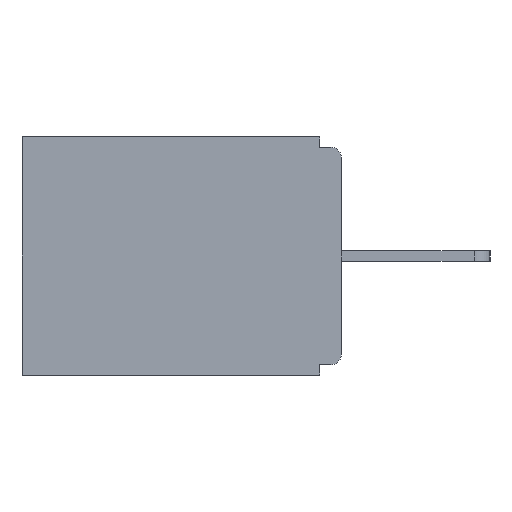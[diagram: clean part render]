
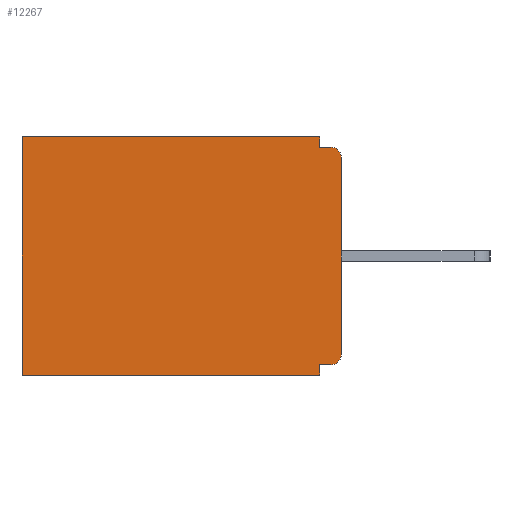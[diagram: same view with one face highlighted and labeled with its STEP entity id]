
A CAD part, left-side view. The second image highlights one B-rep face of the part: STEP entity #12267.
In plain terms, the highlighted planar face has unit normal (-1, 0, 0).
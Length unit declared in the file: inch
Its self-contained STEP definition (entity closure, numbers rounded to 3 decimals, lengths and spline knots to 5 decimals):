
#419 = DIRECTION ( 'NONE',  ( 0., 0., -1. ) ) ;
#435 = EDGE_CURVE ( 'NONE', #12971, #13632, #13769, .T. ) ;
#437 = VERTEX_POINT ( 'NONE', #7959 ) ;
#643 = CARTESIAN_POINT ( 'NONE',  ( 0.298, 0.015, -0.03 ) ) ;
#717 = DIRECTION ( 'NONE',  ( 0., -1., 0. ) ) ;
#756 = VERTEX_POINT ( 'NONE', #13736 ) ;
#789 = CARTESIAN_POINT ( 'NONE',  ( 0.298, 0.031, -0.328 ) ) ;
#1191 = VECTOR ( 'NONE', #7004, 39.37008 ) ;
#1245 = CIRCLE ( 'NONE', #14922, 0.015 ) ;
#1584 = CARTESIAN_POINT ( 'NONE',  ( 0.298, 0., -0.313 ) ) ;
#1650 = LINE ( 'NONE', #3609, #14662 ) ;
#1993 = EDGE_CURVE ( 'NONE', #756, #13632, #1245, .T. ) ;
#2159 = VERTEX_POINT ( 'NONE', #12462 ) ;
#2179 = CARTESIAN_POINT ( 'NONE',  ( 0.298, 0.031, -0.343 ) ) ;
#2371 = DIRECTION ( 'NONE',  ( 0., 1., 0. ) ) ;
#2685 = DIRECTION ( 'NONE',  ( 0., 0., -1. ) ) ;
#2760 = DIRECTION ( 'NONE',  ( -1., 0., 0. ) ) ;
#2870 = FACE_OUTER_BOUND ( 'NONE', #3330, .T. ) ;
#3187 = ORIENTED_EDGE ( 'NONE', *, *, #10290, .F. ) ;
#3330 = EDGE_LOOP ( 'NONE', ( #4592, #10694, #7637, #6819, #8735, #3187, #9320, #3805, #15769, #7374 ) ) ;
#3609 = CARTESIAN_POINT ( 'NONE',  ( 0.298, 0., -0.328 ) ) ;
#3805 = ORIENTED_EDGE ( 'NONE', *, *, #11930, .F. ) ;
#3869 = AXIS2_PLACEMENT_3D ( 'NONE', #14561, #7063, #15812 ) ;
#4266 = CARTESIAN_POINT ( 'NONE',  ( 0.298, 0.031, -0.343 ) ) ;
#4320 = DIRECTION ( 'NONE',  ( 0., 1., 0. ) ) ;
#4351 = VECTOR ( 'NONE', #5552, 39.37008 ) ;
#4395 = CARTESIAN_POINT ( 'NONE',  ( 0.298, 0., 0. ) ) ;
#4445 = CARTESIAN_POINT ( 'NONE',  ( 0.298, 0., -0.343 ) ) ;
#4592 = ORIENTED_EDGE ( 'NONE', *, *, #1993, .T. ) ;
#4597 = CARTESIAN_POINT ( 'NONE',  ( 0.298, 0., -0.015 ) ) ;
#4654 = LINE ( 'NONE', #14625, #1191 ) ;
#4920 = CARTESIAN_POINT ( 'NONE',  ( 0.298, 0.031, -0.343 ) ) ;
#5164 = CARTESIAN_POINT ( 'NONE',  ( 0.298, 0.015, -0.313 ) ) ;
#5245 = EDGE_CURVE ( 'NONE', #437, #15755, #4654, .T. ) ;
#5552 = DIRECTION ( 'NONE',  ( 0., 0., -1. ) ) ;
#5782 = PLANE ( 'NONE',  #3869 ) ;
#5918 = CARTESIAN_POINT ( 'NONE',  ( 0.298, 0.031, -0.015 ) ) ;
#6418 = VERTEX_POINT ( 'NONE', #4920 ) ;
#6627 = EDGE_CURVE ( 'NONE', #9645, #10092, #11172, .T. ) ;
#6661 = CARTESIAN_POINT ( 'NONE',  ( 0.298, 0.46, 0. ) ) ;
#6819 = ORIENTED_EDGE ( 'NONE', *, *, #5245, .T. ) ;
#6906 = LINE ( 'NONE', #4395, #7250 ) ;
#7004 = DIRECTION ( 'NONE',  ( 0., 1., 0. ) ) ;
#7063 = DIRECTION ( 'NONE',  ( 1., 0., 0. ) ) ;
#7250 = VECTOR ( 'NONE', #419, 39.37008 ) ;
#7374 = ORIENTED_EDGE ( 'NONE', *, *, #15871, .F. ) ;
#7637 = ORIENTED_EDGE ( 'NONE', *, *, #15816, .F. ) ;
#7802 = VECTOR ( 'NONE', #2685, 39.37008 ) ;
#7959 = CARTESIAN_POINT ( 'NONE',  ( 0.298, 0.031, 0. ) ) ;
#8181 = LINE ( 'NONE', #2179, #7802 ) ;
#8604 = CARTESIAN_POINT ( 'NONE',  ( 0.298, 0.015, -0.015 ) ) ;
#8735 = ORIENTED_EDGE ( 'NONE', *, *, #13589, .T. ) ;
#9320 = ORIENTED_EDGE ( 'NONE', *, *, #10179, .F. ) ;
#9574 = VECTOR ( 'NONE', #717, 39.37008 ) ;
#9645 = VERTEX_POINT ( 'NONE', #16099 ) ;
#10048 = VERTEX_POINT ( 'NONE', #789 ) ;
#10092 = VERTEX_POINT ( 'NONE', #1584 ) ;
#10179 = EDGE_CURVE ( 'NONE', #10048, #6418, #8181, .T. ) ;
#10290 = EDGE_CURVE ( 'NONE', #6418, #2159, #13309, .T. ) ;
#10694 = ORIENTED_EDGE ( 'NONE', *, *, #435, .F. ) ;
#10926 = CARTESIAN_POINT ( 'NONE',  ( 0.298, 0.46, 0. ) ) ;
#11172 = CIRCLE ( 'NONE', #16240, 0.015 ) ;
#11930 = EDGE_CURVE ( 'NONE', #9645, #10048, #1650, .T. ) ;
#12267 = ADVANCED_FACE ( 'NONE', ( #2870 ), #5782, .F. ) ;
#12388 = LINE ( 'NONE', #10926, #15776 ) ;
#12435 = DIRECTION ( 'NONE',  ( -1., 0., 0. ) ) ;
#12462 = CARTESIAN_POINT ( 'NONE',  ( 0.298, 0.46, -0.343 ) ) ;
#12971 = VERTEX_POINT ( 'NONE', #5918 ) ;
#13309 = LINE ( 'NONE', #4445, #16227 ) ;
#13589 = EDGE_CURVE ( 'NONE', #15755, #2159, #12388, .T. ) ;
#13632 = VERTEX_POINT ( 'NONE', #8604 ) ;
#13736 = CARTESIAN_POINT ( 'NONE',  ( 0.298, 0., -0.03 ) ) ;
#13769 = LINE ( 'NONE', #4597, #9574 ) ;
#14332 = LINE ( 'NONE', #4266, #4351 ) ;
#14561 = CARTESIAN_POINT ( 'NONE',  ( 0.298, 0., 0. ) ) ;
#14625 = CARTESIAN_POINT ( 'NONE',  ( 0.298, 0., 0. ) ) ;
#14662 = VECTOR ( 'NONE', #2371, 39.37008 ) ;
#14677 = DIRECTION ( 'NONE',  ( 0., 0., -1. ) ) ;
#14922 = AXIS2_PLACEMENT_3D ( 'NONE', #643, #12435, #14677 ) ;
#15755 = VERTEX_POINT ( 'NONE', #6661 ) ;
#15769 = ORIENTED_EDGE ( 'NONE', *, *, #6627, .T. ) ;
#15776 = VECTOR ( 'NONE', #16025, 39.37008 ) ;
#15812 = DIRECTION ( 'NONE',  ( 0., 0., -1. ) ) ;
#15816 = EDGE_CURVE ( 'NONE', #437, #12971, #14332, .T. ) ;
#15871 = EDGE_CURVE ( 'NONE', #756, #10092, #6906, .T. ) ;
#16025 = DIRECTION ( 'NONE',  ( 0., 0., -1. ) ) ;
#16085 = DIRECTION ( 'NONE',  ( 0., 0., -1. ) ) ;
#16099 = CARTESIAN_POINT ( 'NONE',  ( 0.298, 0.015, -0.328 ) ) ;
#16227 = VECTOR ( 'NONE', #4320, 39.37008 ) ;
#16240 = AXIS2_PLACEMENT_3D ( 'NONE', #5164, #2760, #16085 ) ;
